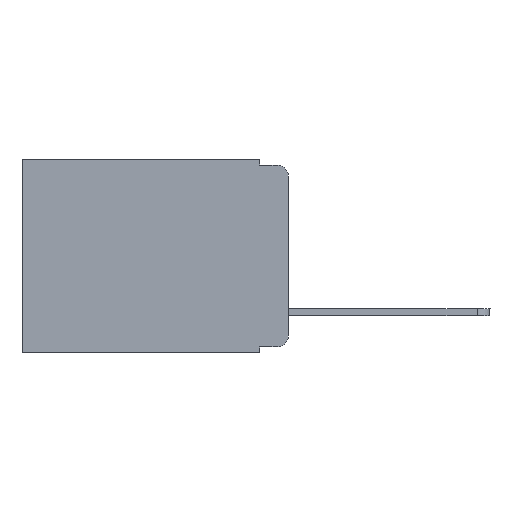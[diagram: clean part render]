
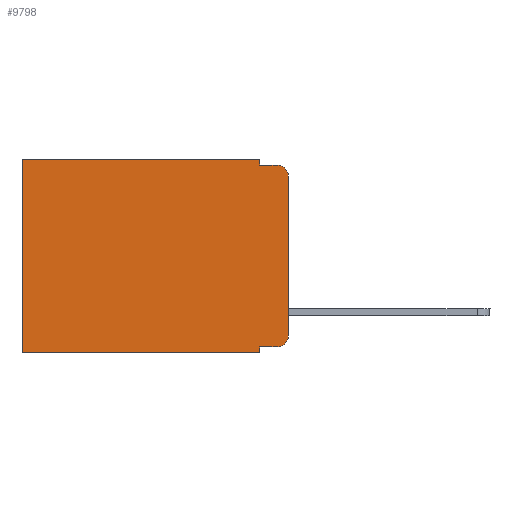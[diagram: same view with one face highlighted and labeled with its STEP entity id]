
A CAD part, left-side view. The second image highlights one B-rep face of the part: STEP entity #9798.
In plain terms, the highlighted planar face has unit normal (-1, 0, 0).
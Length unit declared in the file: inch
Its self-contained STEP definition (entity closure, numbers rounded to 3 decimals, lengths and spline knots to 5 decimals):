
#12 = ORIENTED_EDGE ( 'NONE', *, *, #6170, .F. ) ;
#94 = VECTOR ( 'NONE', #9953, 39.37008 ) ;
#321 = EDGE_CURVE ( 'NONE', #3226, #12572, #3073, .T. ) ;
#458 = CARTESIAN_POINT ( 'NONE',  ( 0.298, 0., 0. ) ) ;
#693 = VECTOR ( 'NONE', #4950, 39.37008 ) ;
#747 = CARTESIAN_POINT ( 'NONE',  ( 0.298, 0.051, -0.333 ) ) ;
#860 = VECTOR ( 'NONE', #2650, 39.37008 ) ;
#1079 = VERTEX_POINT ( 'NONE', #11032 ) ;
#1277 = ORIENTED_EDGE ( 'NONE', *, *, #5455, .F. ) ;
#1509 = LINE ( 'NONE', #458, #9692 ) ;
#1652 = CARTESIAN_POINT ( 'NONE',  ( 0.298, 0.473, 0. ) ) ;
#1670 = LINE ( 'NONE', #10925, #860 ) ;
#1939 = LINE ( 'NONE', #8090, #11121 ) ;
#2006 = ORIENTED_EDGE ( 'NONE', *, *, #5703, .T. ) ;
#2226 = PLANE ( 'NONE',  #6346 ) ;
#2475 = DIRECTION ( 'NONE',  ( 0., 0., -1. ) ) ;
#2650 = DIRECTION ( 'NONE',  ( 0., 1., 0. ) ) ;
#2720 = LINE ( 'NONE', #3720, #693 ) ;
#2860 = VERTEX_POINT ( 'NONE', #5928 ) ;
#3036 = EDGE_CURVE ( 'NONE', #8463, #10819, #11454, .T. ) ;
#3073 = LINE ( 'NONE', #11143, #94 ) ;
#3226 = VERTEX_POINT ( 'NONE', #6442 ) ;
#3390 = VECTOR ( 'NONE', #7814, 39.37008 ) ;
#3451 = DIRECTION ( 'NONE',  ( 0., 0., -1. ) ) ;
#3465 = CARTESIAN_POINT ( 'NONE',  ( 0.298, 0.02, -0.03 ) ) ;
#3520 = ORIENTED_EDGE ( 'NONE', *, *, #9886, .F. ) ;
#3720 = CARTESIAN_POINT ( 'NONE',  ( 0.298, 0.051, 0. ) ) ;
#4142 = CARTESIAN_POINT ( 'NONE',  ( 0.298, 0.051, 0. ) ) ;
#4145 = CARTESIAN_POINT ( 'NONE',  ( 0.298, 0., 0. ) ) ;
#4155 = CARTESIAN_POINT ( 'NONE',  ( 0.298, 0.02, -0.313 ) ) ;
#4385 = LINE ( 'NONE', #12368, #11493 ) ;
#4565 = ORIENTED_EDGE ( 'NONE', *, *, #7940, .T. ) ;
#4741 = LINE ( 'NONE', #747, #3390 ) ;
#4910 = EDGE_CURVE ( 'NONE', #1079, #12572, #11048, .T. ) ;
#4950 = DIRECTION ( 'NONE',  ( 0., 0., -1. ) ) ;
#4955 = DIRECTION ( 'NONE',  ( 0., 0., -1. ) ) ;
#5054 = DIRECTION ( 'NONE',  ( 1., 0., 0. ) ) ;
#5455 = EDGE_CURVE ( 'NONE', #9478, #9589, #4385, .T. ) ;
#5534 = ORIENTED_EDGE ( 'NONE', *, *, #4910, .T. ) ;
#5623 = EDGE_LOOP ( 'NONE', ( #3520, #5534, #7916, #6713, #9594, #2006, #12, #1277, #4565, #6911 ) ) ;
#5703 = EDGE_CURVE ( 'NONE', #6597, #2860, #1939, .T. ) ;
#5928 = CARTESIAN_POINT ( 'NONE',  ( 0.298, 0.473, -0.343 ) ) ;
#6049 = DIRECTION ( 'NONE',  ( 0., 1., 0. ) ) ;
#6170 = EDGE_CURVE ( 'NONE', #9589, #2860, #1670, .T. ) ;
#6346 = AXIS2_PLACEMENT_3D ( 'NONE', #4145, #5054, #12200 ) ;
#6442 = CARTESIAN_POINT ( 'NONE',  ( 0.298, 0.051, -0.01 ) ) ;
#6597 = VERTEX_POINT ( 'NONE', #1652 ) ;
#6713 = ORIENTED_EDGE ( 'NONE', *, *, #7462, .F. ) ;
#6754 = VECTOR ( 'NONE', #6049, 39.37008 ) ;
#6911 = ORIENTED_EDGE ( 'NONE', *, *, #3036, .T. ) ;
#7456 = CARTESIAN_POINT ( 'NONE',  ( 0.298, 0., -0.313 ) ) ;
#7462 = EDGE_CURVE ( 'NONE', #8525, #3226, #2720, .T. ) ;
#7671 = AXIS2_PLACEMENT_3D ( 'NONE', #4155, #9235, #8134 ) ;
#7814 = DIRECTION ( 'NONE',  ( 0., -1., 0. ) ) ;
#7916 = ORIENTED_EDGE ( 'NONE', *, *, #321, .F. ) ;
#7940 = EDGE_CURVE ( 'NONE', #9478, #8463, #4741, .T. ) ;
#8090 = CARTESIAN_POINT ( 'NONE',  ( 0.298, 0.473, 0. ) ) ;
#8134 = DIRECTION ( 'NONE',  ( 0., 0., -1. ) ) ;
#8190 = FACE_OUTER_BOUND ( 'NONE', #5623, .T. ) ;
#8463 = VERTEX_POINT ( 'NONE', #10960 ) ;
#8525 = VERTEX_POINT ( 'NONE', #4142 ) ;
#8584 = CARTESIAN_POINT ( 'NONE',  ( 0.298, 0.051, -0.343 ) ) ;
#9138 = AXIS2_PLACEMENT_3D ( 'NONE', #3465, #9486, #2475 ) ;
#9235 = DIRECTION ( 'NONE',  ( -1., 0., 0. ) ) ;
#9420 = DIRECTION ( 'NONE',  ( 0., 0., -1. ) ) ;
#9456 = CARTESIAN_POINT ( 'NONE',  ( 0.298, 0.02, -0.01 ) ) ;
#9478 = VERTEX_POINT ( 'NONE', #11491 ) ;
#9486 = DIRECTION ( 'NONE',  ( -1., 0., 0. ) ) ;
#9589 = VERTEX_POINT ( 'NONE', #8584 ) ;
#9594 = ORIENTED_EDGE ( 'NONE', *, *, #9713, .T. ) ;
#9692 = VECTOR ( 'NONE', #9420, 39.37008 ) ;
#9713 = EDGE_CURVE ( 'NONE', #8525, #6597, #11750, .T. ) ;
#9798 = ADVANCED_FACE ( 'NONE', ( #8190 ), #2226, .F. ) ;
#9886 = EDGE_CURVE ( 'NONE', #1079, #10819, #1509, .T. ) ;
#9953 = DIRECTION ( 'NONE',  ( 0., -1., 0. ) ) ;
#10770 = CARTESIAN_POINT ( 'NONE',  ( 0.298, 0., 0. ) ) ;
#10819 = VERTEX_POINT ( 'NONE', #7456 ) ;
#10925 = CARTESIAN_POINT ( 'NONE',  ( 0.298, 0., -0.343 ) ) ;
#10960 = CARTESIAN_POINT ( 'NONE',  ( 0.298, 0.02, -0.333 ) ) ;
#11032 = CARTESIAN_POINT ( 'NONE',  ( 0.298, 0., -0.03 ) ) ;
#11048 = CIRCLE ( 'NONE', #9138, 0.02 ) ;
#11121 = VECTOR ( 'NONE', #4955, 39.37008 ) ;
#11143 = CARTESIAN_POINT ( 'NONE',  ( 0.298, 0.051, -0.01 ) ) ;
#11454 = CIRCLE ( 'NONE', #7671, 0.02 ) ;
#11491 = CARTESIAN_POINT ( 'NONE',  ( 0.298, 0.051, -0.333 ) ) ;
#11493 = VECTOR ( 'NONE', #3451, 39.37008 ) ;
#11750 = LINE ( 'NONE', #10770, #6754 ) ;
#12200 = DIRECTION ( 'NONE',  ( 0., 0., -1. ) ) ;
#12368 = CARTESIAN_POINT ( 'NONE',  ( 0.298, 0.051, 0. ) ) ;
#12572 = VERTEX_POINT ( 'NONE', #9456 ) ;
